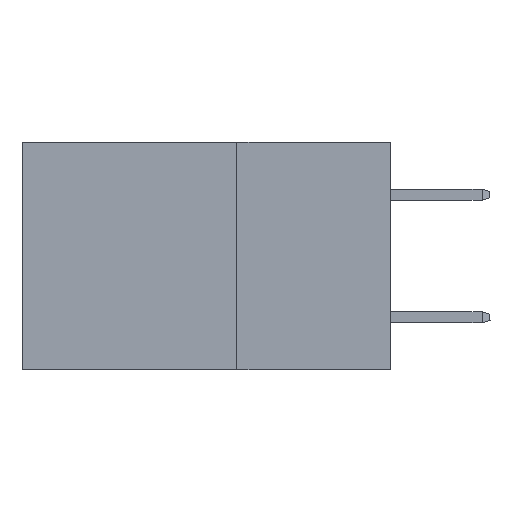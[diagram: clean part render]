
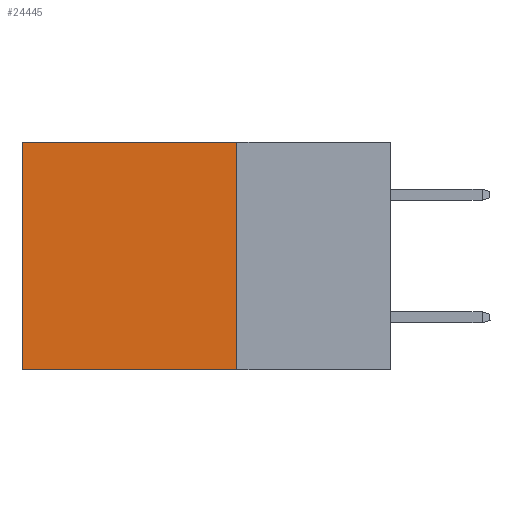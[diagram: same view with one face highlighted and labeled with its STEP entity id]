
A CAD part, left-side view. The second image highlights one B-rep face of the part: STEP entity #24445.
In plain terms, the highlighted planar face has unit normal (-1, 0, 0).
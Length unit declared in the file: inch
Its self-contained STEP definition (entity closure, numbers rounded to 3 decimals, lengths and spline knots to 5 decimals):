
#263 = CARTESIAN_POINT ( 'NONE',  ( 0.2875, 0.25, -0.37 ) ) ;
#1392 = CARTESIAN_POINT ( 'NONE',  ( 0.2875, 0.6, -0.37 ) ) ;
#1495 = CARTESIAN_POINT ( 'NONE',  ( 0.2875, 0.25, 0. ) ) ;
#1736 = VERTEX_POINT ( 'NONE', #15749 ) ;
#2215 = FACE_OUTER_BOUND ( 'NONE', #5738, .T. ) ;
#5738 = EDGE_LOOP ( 'NONE', ( #25918, #11351, #13858, #19675 ) ) ;
#5839 = PLANE ( 'NONE',  #10683 ) ;
#7470 = VERTEX_POINT ( 'NONE', #1392 ) ;
#8374 = DIRECTION ( 'NONE',  ( 0., 1., 0. ) ) ;
#9173 = VECTOR ( 'NONE', #12256, 39.37008 ) ;
#9743 = DIRECTION ( 'NONE',  ( 0., 0., -1. ) ) ;
#9891 = CARTESIAN_POINT ( 'NONE',  ( 0.2875, 0.6, 0. ) ) ;
#10408 = VECTOR ( 'NONE', #16075, 39.37008 ) ;
#10635 = VERTEX_POINT ( 'NONE', #11994 ) ;
#10683 = AXIS2_PLACEMENT_3D ( 'NONE', #20698, #22339, #16106 ) ;
#11351 = ORIENTED_EDGE ( 'NONE', *, *, #16698, .F. ) ;
#11994 = CARTESIAN_POINT ( 'NONE',  ( 0.2875, 0.6, 0. ) ) ;
#12256 = DIRECTION ( 'NONE',  ( 0., 0., -1. ) ) ;
#12978 = EDGE_CURVE ( 'NONE', #1736, #16012, #21567, .T. ) ;
#13079 = EDGE_CURVE ( 'NONE', #1736, #10635, #15332, .T. ) ;
#13858 = ORIENTED_EDGE ( 'NONE', *, *, #12978, .F. ) ;
#15332 = LINE ( 'NONE', #1495, #10408 ) ;
#15749 = CARTESIAN_POINT ( 'NONE',  ( 0.2875, 0.25, 0. ) ) ;
#16012 = VERTEX_POINT ( 'NONE', #263 ) ;
#16075 = DIRECTION ( 'NONE',  ( 0., 1., 0. ) ) ;
#16106 = DIRECTION ( 'NONE',  ( 0., 0., -1. ) ) ;
#16283 = VECTOR ( 'NONE', #8374, 39.37008 ) ;
#16698 = EDGE_CURVE ( 'NONE', #16012, #7470, #20563, .T. ) ;
#19010 = CARTESIAN_POINT ( 'NONE',  ( 0.2875, 0.25, -0.37 ) ) ;
#19675 = ORIENTED_EDGE ( 'NONE', *, *, #13079, .T. ) ;
#20563 = LINE ( 'NONE', #19010, #16283 ) ;
#20698 = CARTESIAN_POINT ( 'NONE',  ( 0.2875, 0.25, 0. ) ) ;
#20826 = EDGE_CURVE ( 'NONE', #10635, #7470, #26968, .T. ) ;
#21567 = LINE ( 'NONE', #24626, #25887 ) ;
#22339 = DIRECTION ( 'NONE',  ( 1., 0., 0. ) ) ;
#24445 = ADVANCED_FACE ( 'NONE', ( #2215 ), #5839, .F. ) ;
#24626 = CARTESIAN_POINT ( 'NONE',  ( 0.2875, 0.25, 0. ) ) ;
#25887 = VECTOR ( 'NONE', #9743, 39.37008 ) ;
#25918 = ORIENTED_EDGE ( 'NONE', *, *, #20826, .T. ) ;
#26968 = LINE ( 'NONE', #9891, #9173 ) ;
